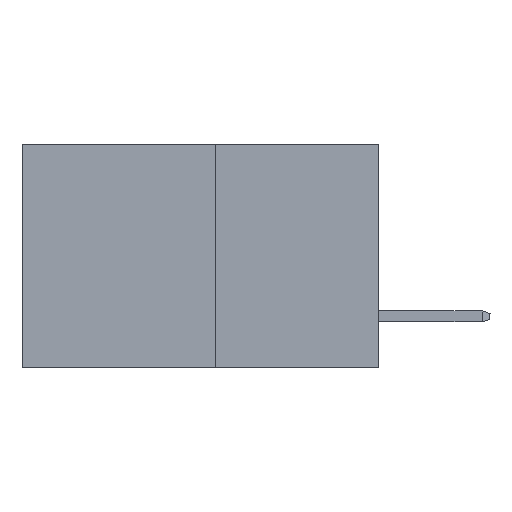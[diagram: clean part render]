
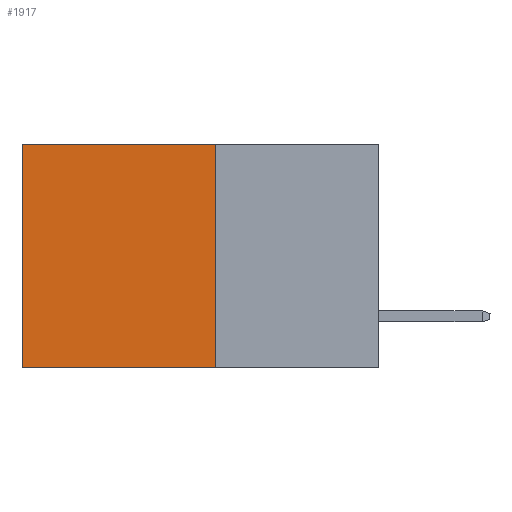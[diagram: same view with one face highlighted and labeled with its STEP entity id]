
A CAD part, left-side view. The second image highlights one B-rep face of the part: STEP entity #1917.
In plain terms, the highlighted planar face has unit normal (-1, 0, 0).
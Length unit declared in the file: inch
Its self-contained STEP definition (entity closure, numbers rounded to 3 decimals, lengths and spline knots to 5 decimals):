
#195 = DIRECTION ( 'NONE',  ( 0., 0., -1. ) ) ;
#213 = DIRECTION ( 'NONE',  ( 1., 0., 0. ) ) ;
#278 = ORIENTED_EDGE ( 'NONE', *, *, #11345, .F. ) ;
#297 = CARTESIAN_POINT ( 'NONE',  ( 0.277, 0.27, -0.37 ) ) ;
#298 = VERTEX_POINT ( 'NONE', #6485 ) ;
#362 = DIRECTION ( 'NONE',  ( 0., 1., 0. ) ) ;
#718 = CARTESIAN_POINT ( 'NONE',  ( 0.277, 0.59, -0.37 ) ) ;
#1402 = PLANE ( 'NONE',  #3740 ) ;
#1917 = ADVANCED_FACE ( 'NONE', ( #12159 ), #1402, .F. ) ;
#2098 = CARTESIAN_POINT ( 'NONE',  ( 0.277, 0.27, -0.37 ) ) ;
#2810 = CARTESIAN_POINT ( 'NONE',  ( 0.277, 0.59, -0.37 ) ) ;
#2882 = EDGE_CURVE ( 'NONE', #8727, #298, #11868, .T. ) ;
#3072 = VECTOR ( 'NONE', #9141, 39.37008 ) ;
#3110 = DIRECTION ( 'NONE',  ( 0., 0., -1. ) ) ;
#3360 = ORIENTED_EDGE ( 'NONE', *, *, #2882, .T. ) ;
#3379 = CARTESIAN_POINT ( 'NONE',  ( 0.277, 0.27, -0.37 ) ) ;
#3740 = AXIS2_PLACEMENT_3D ( 'NONE', #297, #213, #195 ) ;
#4266 = EDGE_LOOP ( 'NONE', ( #4771, #278, #10363, #3360 ) ) ;
#4613 = CARTESIAN_POINT ( 'NONE',  ( 0.277, 0.27, -0.37 ) ) ;
#4771 = ORIENTED_EDGE ( 'NONE', *, *, #7431, .T. ) ;
#5741 = DIRECTION ( 'NONE',  ( 0., 0., -1. ) ) ;
#6088 = VERTEX_POINT ( 'NONE', #718 ) ;
#6173 = LINE ( 'NONE', #2810, #8309 ) ;
#6485 = CARTESIAN_POINT ( 'NONE',  ( 0.277, 0.59, 0. ) ) ;
#7431 = EDGE_CURVE ( 'NONE', #298, #6088, #6173, .T. ) ;
#7682 = VECTOR ( 'NONE', #3110, 39.37008 ) ;
#8309 = VECTOR ( 'NONE', #5741, 39.37008 ) ;
#8410 = VERTEX_POINT ( 'NONE', #3379 ) ;
#8515 = LINE ( 'NONE', #2098, #7682 ) ;
#8727 = VERTEX_POINT ( 'NONE', #9581 ) ;
#9141 = DIRECTION ( 'NONE',  ( 0., 1., 0. ) ) ;
#9581 = CARTESIAN_POINT ( 'NONE',  ( 0.277, 0.27, 0. ) ) ;
#10031 = EDGE_CURVE ( 'NONE', #8727, #8410, #8515, .T. ) ;
#10067 = VECTOR ( 'NONE', #362, 39.37008 ) ;
#10148 = LINE ( 'NONE', #4613, #3072 ) ;
#10234 = CARTESIAN_POINT ( 'NONE',  ( 0.277, 0.27, 0. ) ) ;
#10363 = ORIENTED_EDGE ( 'NONE', *, *, #10031, .F. ) ;
#11345 = EDGE_CURVE ( 'NONE', #8410, #6088, #10148, .T. ) ;
#11868 = LINE ( 'NONE', #10234, #10067 ) ;
#12159 = FACE_OUTER_BOUND ( 'NONE', #4266, .T. ) ;
